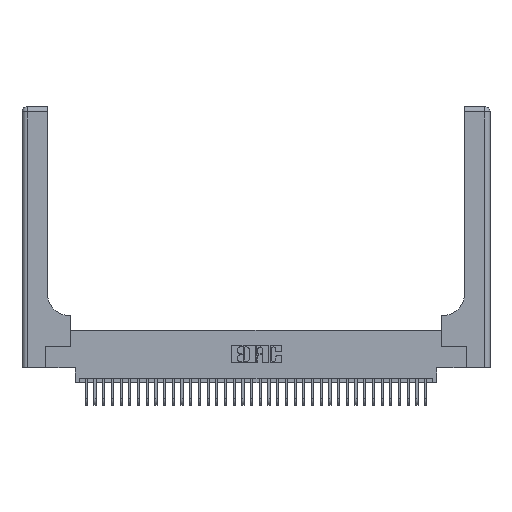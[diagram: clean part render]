
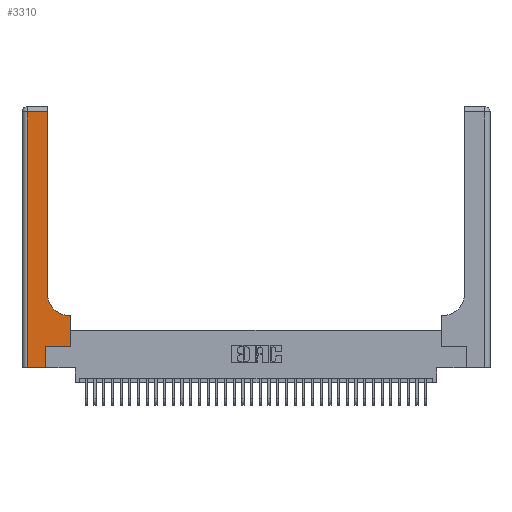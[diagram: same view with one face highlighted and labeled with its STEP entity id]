
A CAD part, top view. The second image highlights one B-rep face of the part: STEP entity #3310.
In plain terms, the highlighted planar face has unit normal (0, 0, 1).
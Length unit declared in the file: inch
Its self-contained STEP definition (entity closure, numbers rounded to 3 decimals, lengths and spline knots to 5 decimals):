
#269 = DIRECTION ( 'NONE',  ( -1., 0., 0. ) ) ;
#374 = VECTOR ( 'NONE', #32196, 39.37008 ) ;
#1212 = EDGE_CURVE ( 'NONE', #19815, #35833, #3712, .T. ) ;
#1390 = CARTESIAN_POINT ( 'NONE',  ( 0.2915, 3., 0.37 ) ) ;
#2840 = CARTESIAN_POINT ( 'NONE',  ( 0.269, 0.25, 0.37 ) ) ;
#3101 = LINE ( 'NONE', #1390, #16446 ) ;
#3178 = CARTESIAN_POINT ( 'NONE',  ( 0., 0., 0.37 ) ) ;
#3310 = ADVANCED_FACE ( 'NONE', ( #3612 ), #36089, .F. ) ;
#3466 = DIRECTION ( 'NONE',  ( -1., 0., 0. ) ) ;
#3612 = FACE_OUTER_BOUND ( 'NONE', #31116, .T. ) ;
#3712 = CIRCLE ( 'NONE', #9568, 0.25 ) ;
#5205 = LINE ( 'NONE', #3178, #19387 ) ;
#5768 = ORIENTED_EDGE ( 'NONE', *, *, #17197, .T. ) ;
#6392 = DIRECTION ( 'NONE',  ( 0., 0., -1. ) ) ;
#7127 = VECTOR ( 'NONE', #26799, 39.37008 ) ;
#8659 = CARTESIAN_POINT ( 'NONE',  ( 0.06, 0., 0.37 ) ) ;
#9568 = AXIS2_PLACEMENT_3D ( 'NONE', #24360, #6392, #27286 ) ;
#9814 = VECTOR ( 'NONE', #3466, 39.37008 ) ;
#9876 = VERTEX_POINT ( 'NONE', #32091 ) ;
#10415 = ORIENTED_EDGE ( 'NONE', *, *, #14243, .T. ) ;
#10956 = VERTEX_POINT ( 'NONE', #29031 ) ;
#11376 = LINE ( 'NONE', #2840, #12344 ) ;
#11388 = CARTESIAN_POINT ( 'NONE',  ( 0.06, 3., 0.37 ) ) ;
#11885 = ORIENTED_EDGE ( 'NONE', *, *, #1212, .T. ) ;
#12344 = VECTOR ( 'NONE', #23968, 39.37008 ) ;
#12532 = VECTOR ( 'NONE', #15746, 39.37008 ) ;
#12944 = VERTEX_POINT ( 'NONE', #26762 ) ;
#13417 = CARTESIAN_POINT ( 'NONE',  ( 0.269, 0., 0.37 ) ) ;
#14243 = EDGE_CURVE ( 'NONE', #36064, #14852, #24501, .T. ) ;
#14852 = VERTEX_POINT ( 'NONE', #8659 ) ;
#14872 = CARTESIAN_POINT ( 'NONE',  ( 0., 2.94, 0.37 ) ) ;
#15513 = CARTESIAN_POINT ( 'NONE',  ( 0., 3., 0.37 ) ) ;
#15528 = CARTESIAN_POINT ( 'NONE',  ( 0.5585, 0.25, 0.37 ) ) ;
#15606 = CARTESIAN_POINT ( 'NONE',  ( 0.2915, 0.6, 0.37 ) ) ;
#15746 = DIRECTION ( 'NONE',  ( 0., 1., 0. ) ) ;
#16446 = VECTOR ( 'NONE', #28310, 39.37008 ) ;
#17197 = EDGE_CURVE ( 'NONE', #12944, #9876, #30228, .T. ) ;
#17464 = ORIENTED_EDGE ( 'NONE', *, *, #26283, .T. ) ;
#17880 = LINE ( 'NONE', #15606, #9814 ) ;
#18525 = DIRECTION ( 'NONE',  ( 0., 0., -1. ) ) ;
#18628 = CARTESIAN_POINT ( 'NONE',  ( 0.5585, 0.25, 0.37 ) ) ;
#19065 = ORIENTED_EDGE ( 'NONE', *, *, #25377, .T. ) ;
#19387 = VECTOR ( 'NONE', #27214, 39.37008 ) ;
#19576 = EDGE_CURVE ( 'NONE', #19919, #36064, #24026, .T. ) ;
#19815 = VERTEX_POINT ( 'NONE', #27795 ) ;
#19919 = VERTEX_POINT ( 'NONE', #33930 ) ;
#19976 = ORIENTED_EDGE ( 'NONE', *, *, #29299, .T. ) ;
#21406 = ORIENTED_EDGE ( 'NONE', *, *, #27291, .T. ) ;
#21944 = VERTEX_POINT ( 'NONE', #15528 ) ;
#23968 = DIRECTION ( 'NONE',  ( 1., 0., 0. ) ) ;
#24026 = LINE ( 'NONE', #14872, #7127 ) ;
#24360 = CARTESIAN_POINT ( 'NONE',  ( 0.5415, 0.85, 0.37 ) ) ;
#24501 = LINE ( 'NONE', #11388, #374 ) ;
#25342 = ORIENTED_EDGE ( 'NONE', *, *, #19576, .T. ) ;
#25377 = EDGE_CURVE ( 'NONE', #10956, #19815, #17880, .T. ) ;
#26283 = EDGE_CURVE ( 'NONE', #35833, #19919, #3101, .T. ) ;
#26762 = CARTESIAN_POINT ( 'NONE',  ( 0.269, 0., 0.37 ) ) ;
#26799 = DIRECTION ( 'NONE',  ( -1., 0., 0. ) ) ;
#27214 = DIRECTION ( 'NONE',  ( 1., 0., 0. ) ) ;
#27286 = DIRECTION ( 'NONE',  ( 1., 0., 0. ) ) ;
#27291 = EDGE_CURVE ( 'NONE', #21944, #10956, #29259, .T. ) ;
#27795 = CARTESIAN_POINT ( 'NONE',  ( 0.5415, 0.6, 0.37 ) ) ;
#28310 = DIRECTION ( 'NONE',  ( 0., 1., 0. ) ) ;
#29031 = CARTESIAN_POINT ( 'NONE',  ( 0.5585, 0.6, 0.37 ) ) ;
#29259 = LINE ( 'NONE', #18628, #12532 ) ;
#29291 = VECTOR ( 'NONE', #31175, 39.37008 ) ;
#29299 = EDGE_CURVE ( 'NONE', #9876, #21944, #11376, .T. ) ;
#30228 = LINE ( 'NONE', #13417, #29291 ) ;
#30809 = CARTESIAN_POINT ( 'NONE',  ( 0.06, 2.94, 0.37 ) ) ;
#31116 = EDGE_LOOP ( 'NONE', ( #17464, #25342, #10415, #35949, #5768, #19976, #21406, #19065, #11885 ) ) ;
#31175 = DIRECTION ( 'NONE',  ( 0., 1., 0. ) ) ;
#32091 = CARTESIAN_POINT ( 'NONE',  ( 0.269, 0.25, 0.37 ) ) ;
#32196 = DIRECTION ( 'NONE',  ( 0., -1., 0. ) ) ;
#33701 = AXIS2_PLACEMENT_3D ( 'NONE', #15513, #18525, #269 ) ;
#33930 = CARTESIAN_POINT ( 'NONE',  ( 0.2915, 2.94, 0.37 ) ) ;
#34286 = EDGE_CURVE ( 'NONE', #14852, #12944, #5205, .T. ) ;
#35035 = CARTESIAN_POINT ( 'NONE',  ( 0.2915, 0.85, 0.37 ) ) ;
#35833 = VERTEX_POINT ( 'NONE', #35035 ) ;
#35949 = ORIENTED_EDGE ( 'NONE', *, *, #34286, .T. ) ;
#36064 = VERTEX_POINT ( 'NONE', #30809 ) ;
#36089 = PLANE ( 'NONE',  #33701 ) ;
